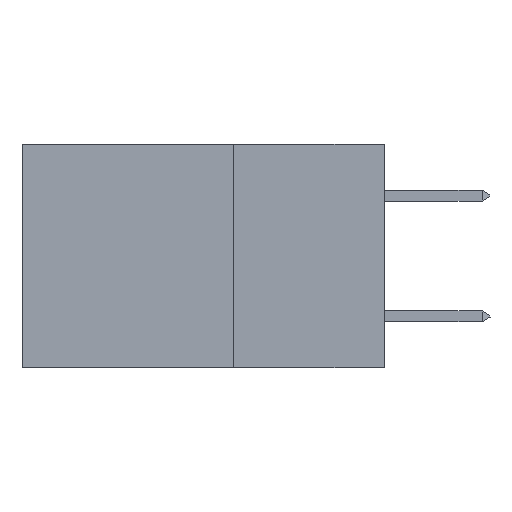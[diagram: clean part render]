
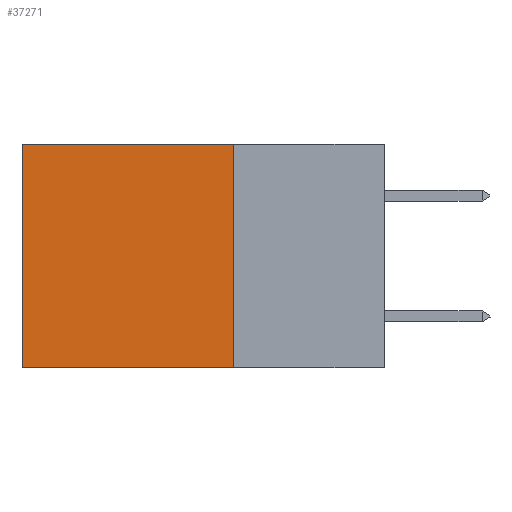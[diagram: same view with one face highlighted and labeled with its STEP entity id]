
A CAD part, left-side view. The second image highlights one B-rep face of the part: STEP entity #37271.
In plain terms, the highlighted planar face has unit normal (-1, 0, 0).
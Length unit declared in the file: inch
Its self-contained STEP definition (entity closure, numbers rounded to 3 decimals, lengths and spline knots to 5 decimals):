
#326 = EDGE_CURVE ( 'NONE', #45082, #23087, #22296, .T. ) ;
#740 = EDGE_CURVE ( 'NONE', #1924, #23087, #29737, .T. ) ;
#787 = ORIENTED_EDGE ( 'NONE', *, *, #36266, .F. ) ;
#1861 = VERTEX_POINT ( 'NONE', #7833 ) ;
#1924 = VERTEX_POINT ( 'NONE', #38977 ) ;
#4763 = DIRECTION ( 'NONE',  ( 1., 0., 0. ) ) ;
#7833 = CARTESIAN_POINT ( 'NONE',  ( 0.2875, 0.25, 0. ) ) ;
#8996 = LINE ( 'NONE', #29381, #28912 ) ;
#9512 = CARTESIAN_POINT ( 'NONE',  ( 0.2875, 0.6, -0.37 ) ) ;
#10232 = VECTOR ( 'NONE', #36708, 39.37008 ) ;
#15034 = CARTESIAN_POINT ( 'NONE',  ( 0.2875, 0.25, 0. ) ) ;
#15044 = ORIENTED_EDGE ( 'NONE', *, *, #22930, .T. ) ;
#16227 = DIRECTION ( 'NONE',  ( 0., 1., 0. ) ) ;
#18738 = DIRECTION ( 'NONE',  ( 0., 0., -1. ) ) ;
#18758 = AXIS2_PLACEMENT_3D ( 'NONE', #32692, #4763, #18738 ) ;
#19538 = ORIENTED_EDGE ( 'NONE', *, *, #326, .T. ) ;
#19889 = CARTESIAN_POINT ( 'NONE',  ( 0.2875, 0.25, -0.37 ) ) ;
#21600 = ORIENTED_EDGE ( 'NONE', *, *, #740, .F. ) ;
#22172 = FACE_OUTER_BOUND ( 'NONE', #23940, .T. ) ;
#22296 = LINE ( 'NONE', #40144, #10232 ) ;
#22305 = VECTOR ( 'NONE', #43418, 39.37008 ) ;
#22930 = EDGE_CURVE ( 'NONE', #1861, #45082, #25111, .T. ) ;
#23087 = VERTEX_POINT ( 'NONE', #9512 ) ;
#23940 = EDGE_LOOP ( 'NONE', ( #19538, #21600, #787, #15044 ) ) ;
#24975 = CARTESIAN_POINT ( 'NONE',  ( 0.2875, 0.6, 0. ) ) ;
#25111 = LINE ( 'NONE', #15034, #22305 ) ;
#28912 = VECTOR ( 'NONE', #29824, 39.37008 ) ;
#29381 = CARTESIAN_POINT ( 'NONE',  ( 0.2875, 0.25, 0. ) ) ;
#29737 = LINE ( 'NONE', #19889, #35850 ) ;
#29824 = DIRECTION ( 'NONE',  ( 0., 0., -1. ) ) ;
#32692 = CARTESIAN_POINT ( 'NONE',  ( 0.2875, 0.25, 0. ) ) ;
#35850 = VECTOR ( 'NONE', #16227, 39.37008 ) ;
#36266 = EDGE_CURVE ( 'NONE', #1861, #1924, #8996, .T. ) ;
#36708 = DIRECTION ( 'NONE',  ( 0., 0., -1. ) ) ;
#37271 = ADVANCED_FACE ( 'NONE', ( #22172 ), #43004, .F. ) ;
#38977 = CARTESIAN_POINT ( 'NONE',  ( 0.2875, 0.25, -0.37 ) ) ;
#40144 = CARTESIAN_POINT ( 'NONE',  ( 0.2875, 0.6, 0. ) ) ;
#43004 = PLANE ( 'NONE',  #18758 ) ;
#43418 = DIRECTION ( 'NONE',  ( 0., 1., 0. ) ) ;
#45082 = VERTEX_POINT ( 'NONE', #24975 ) ;
